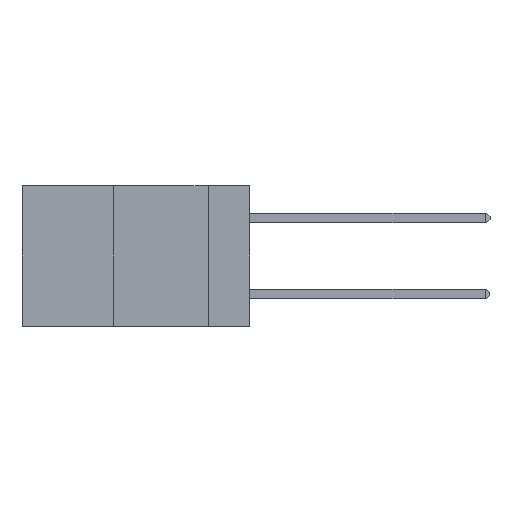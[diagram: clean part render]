
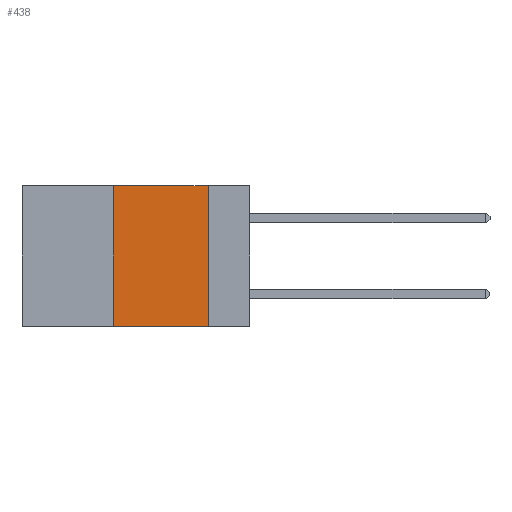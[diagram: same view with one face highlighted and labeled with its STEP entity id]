
A CAD part, left-side view. The second image highlights one B-rep face of the part: STEP entity #438.
In plain terms, the highlighted planar face has unit normal (-1, 0, 0).
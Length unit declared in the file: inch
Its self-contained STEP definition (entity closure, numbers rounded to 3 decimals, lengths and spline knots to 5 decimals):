
#122 = EDGE_LOOP ( 'NONE', ( #715, #724, #784, #862 ) ) ;
#405 = DIRECTION ( 'NONE',  ( 0., -1., 0. ) ) ;
#423 = VECTOR ( 'NONE', #9934, 39.37008 ) ;
#438 = ADVANCED_FACE ( 'NONE', ( #3312 ), #2768, .F. ) ;
#715 = ORIENTED_EDGE ( 'NONE', *, *, #1963, .F. ) ;
#724 = ORIENTED_EDGE ( 'NONE', *, *, #7310, .F. ) ;
#784 = ORIENTED_EDGE ( 'NONE', *, *, #9342, .F. ) ;
#862 = ORIENTED_EDGE ( 'NONE', *, *, #1599, .T. ) ;
#941 = VERTEX_POINT ( 'NONE', #3467 ) ;
#1512 = VERTEX_POINT ( 'NONE', #1802 ) ;
#1599 = EDGE_CURVE ( 'NONE', #8491, #941, #8032, .T. ) ;
#1802 = CARTESIAN_POINT ( 'NONE',  ( 0., 0.11, 0. ) ) ;
#1963 = EDGE_CURVE ( 'NONE', #1512, #941, #2872, .T. ) ;
#2030 = CARTESIAN_POINT ( 'NONE',  ( 0., 0.36, -0.37 ) ) ;
#2299 = CARTESIAN_POINT ( 'NONE',  ( 0., 0.36, 0. ) ) ;
#2350 = DIRECTION ( 'NONE',  ( 1., 0., 0. ) ) ;
#2765 = DIRECTION ( 'NONE',  ( 0., -1., 0. ) ) ;
#2768 = PLANE ( 'NONE',  #5900 ) ;
#2872 = LINE ( 'NONE', #9995, #423 ) ;
#3157 = DIRECTION ( 'NONE',  ( 0., 0., 1. ) ) ;
#3312 = FACE_OUTER_BOUND ( 'NONE', #122, .T. ) ;
#3467 = CARTESIAN_POINT ( 'NONE',  ( 0., 0.11, -0.37 ) ) ;
#3681 = LINE ( 'NONE', #2299, #5490 ) ;
#4076 = VECTOR ( 'NONE', #2765, 39.37008 ) ;
#4544 = DIRECTION ( 'NONE',  ( 0., 0., -1. ) ) ;
#4859 = CARTESIAN_POINT ( 'NONE',  ( 0., 0.6, 0. ) ) ;
#4983 = CARTESIAN_POINT ( 'NONE',  ( 0., 0.6, -0.37 ) ) ;
#5490 = VECTOR ( 'NONE', #3157, 39.37008 ) ;
#5900 = AXIS2_PLACEMENT_3D ( 'NONE', #4859, #2350, #4544 ) ;
#7310 = EDGE_CURVE ( 'NONE', #8247, #1512, #8242, .T. ) ;
#8032 = LINE ( 'NONE', #4983, #4076 ) ;
#8055 = VECTOR ( 'NONE', #405, 39.37008 ) ;
#8242 = LINE ( 'NONE', #9835, #8055 ) ;
#8247 = VERTEX_POINT ( 'NONE', #10105 ) ;
#8491 = VERTEX_POINT ( 'NONE', #2030 ) ;
#9342 = EDGE_CURVE ( 'NONE', #8491, #8247, #3681, .T. ) ;
#9835 = CARTESIAN_POINT ( 'NONE',  ( 0., 0.6, 0. ) ) ;
#9934 = DIRECTION ( 'NONE',  ( 0., 0., -1. ) ) ;
#9995 = CARTESIAN_POINT ( 'NONE',  ( 0., 0.11, 0. ) ) ;
#10105 = CARTESIAN_POINT ( 'NONE',  ( 0., 0.36, 0. ) ) ;
